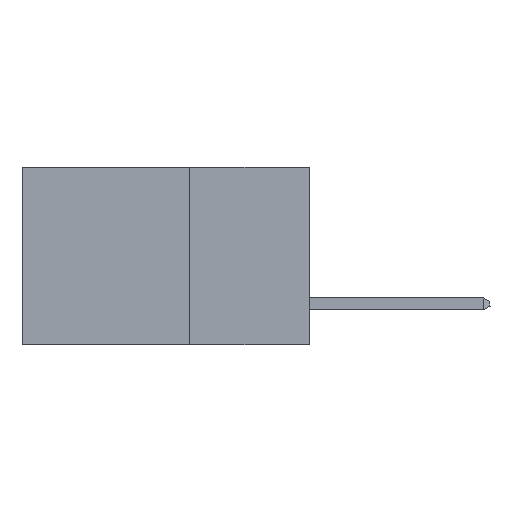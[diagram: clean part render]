
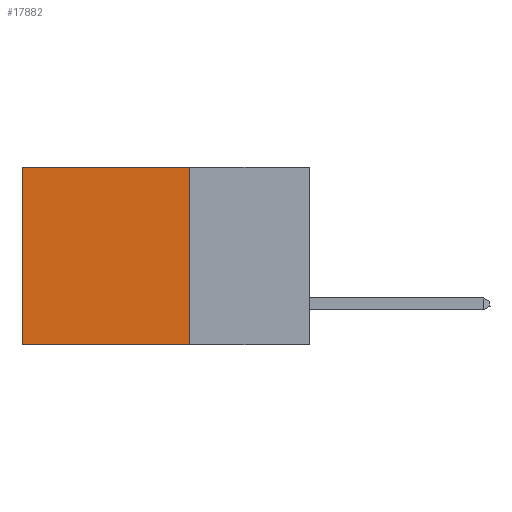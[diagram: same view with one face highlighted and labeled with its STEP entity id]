
A CAD part, left-side view. The second image highlights one B-rep face of the part: STEP entity #17882.
In plain terms, the highlighted planar face has unit normal (-1, 0, 0).
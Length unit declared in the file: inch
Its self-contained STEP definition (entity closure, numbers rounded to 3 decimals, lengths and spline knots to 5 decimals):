
#921 = EDGE_LOOP ( 'NONE', ( #7295, #16424, #27096, #16144 ) ) ;
#3079 = LINE ( 'NONE', #23905, #17481 ) ;
#3204 = CARTESIAN_POINT ( 'NONE',  ( 0.2875, 0.6, 0. ) ) ;
#3770 = VERTEX_POINT ( 'NONE', #21738 ) ;
#3877 = DIRECTION ( 'NONE',  ( 1., 0., 0. ) ) ;
#3944 = EDGE_CURVE ( 'NONE', #5802, #4545, #20250, .T. ) ;
#4545 = VERTEX_POINT ( 'NONE', #5201 ) ;
#4628 = VECTOR ( 'NONE', #27236, 39.37008 ) ;
#4938 = DIRECTION ( 'NONE',  ( 0., 1., 0. ) ) ;
#5201 = CARTESIAN_POINT ( 'NONE',  ( 0.2875, 0.6, -0.37 ) ) ;
#5734 = AXIS2_PLACEMENT_3D ( 'NONE', #11794, #3877, #19454 ) ;
#5802 = VERTEX_POINT ( 'NONE', #32005 ) ;
#7295 = ORIENTED_EDGE ( 'NONE', *, *, #7714, .T. ) ;
#7714 = EDGE_CURVE ( 'NONE', #8088, #4545, #18250, .T. ) ;
#8088 = VERTEX_POINT ( 'NONE', #8807 ) ;
#8807 = CARTESIAN_POINT ( 'NONE',  ( 0.2875, 0.6, 0. ) ) ;
#11794 = CARTESIAN_POINT ( 'NONE',  ( 0.2875, 0.25, 0. ) ) ;
#12789 = EDGE_CURVE ( 'NONE', #3770, #5802, #3079, .T. ) ;
#14885 = FACE_OUTER_BOUND ( 'NONE', #921, .T. ) ;
#16144 = ORIENTED_EDGE ( 'NONE', *, *, #30683, .T. ) ;
#16424 = ORIENTED_EDGE ( 'NONE', *, *, #3944, .F. ) ;
#17481 = VECTOR ( 'NONE', #31940, 39.37008 ) ;
#17743 = VECTOR ( 'NONE', #4938, 39.37008 ) ;
#17882 = ADVANCED_FACE ( 'NONE', ( #14885 ), #18967, .F. ) ;
#18250 = LINE ( 'NONE', #3204, #4628 ) ;
#18967 = PLANE ( 'NONE',  #5734 ) ;
#19454 = DIRECTION ( 'NONE',  ( 0., 0., -1. ) ) ;
#19745 = CARTESIAN_POINT ( 'NONE',  ( 0.2875, 0.25, 0. ) ) ;
#20250 = LINE ( 'NONE', #31193, #17743 ) ;
#21738 = CARTESIAN_POINT ( 'NONE',  ( 0.2875, 0.25, 0. ) ) ;
#23905 = CARTESIAN_POINT ( 'NONE',  ( 0.2875, 0.25, 0. ) ) ;
#24827 = DIRECTION ( 'NONE',  ( 0., 1., 0. ) ) ;
#26126 = LINE ( 'NONE', #19745, #29381 ) ;
#27096 = ORIENTED_EDGE ( 'NONE', *, *, #12789, .F. ) ;
#27236 = DIRECTION ( 'NONE',  ( 0., 0., -1. ) ) ;
#29381 = VECTOR ( 'NONE', #24827, 39.37008 ) ;
#30683 = EDGE_CURVE ( 'NONE', #3770, #8088, #26126, .T. ) ;
#31193 = CARTESIAN_POINT ( 'NONE',  ( 0.2875, 0.25, -0.37 ) ) ;
#31940 = DIRECTION ( 'NONE',  ( 0., 0., -1. ) ) ;
#32005 = CARTESIAN_POINT ( 'NONE',  ( 0.2875, 0.25, -0.37 ) ) ;
